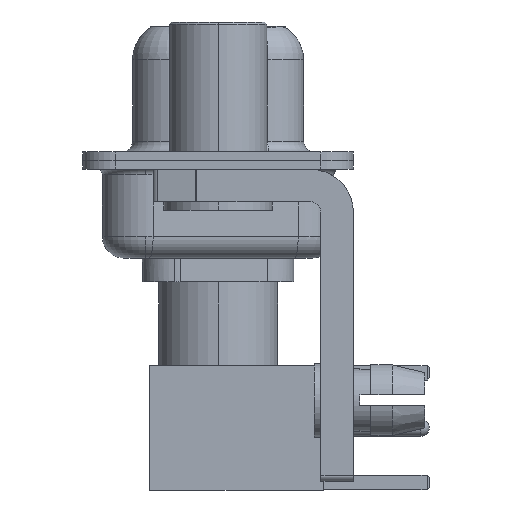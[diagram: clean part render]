
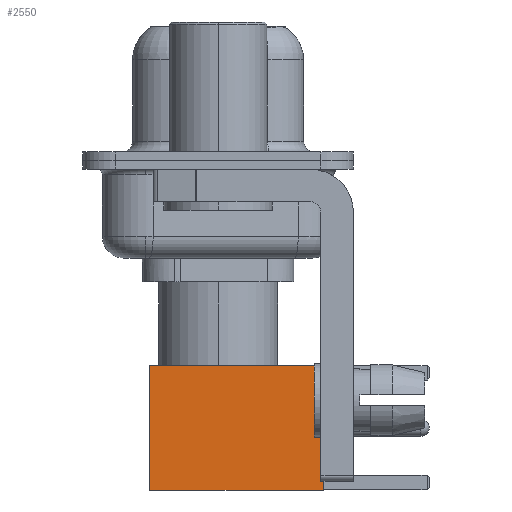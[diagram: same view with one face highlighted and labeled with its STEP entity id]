
A CAD part, left-side view. The second image highlights one B-rep face of the part: STEP entity #2550.
In plain terms, the highlighted face is planar.
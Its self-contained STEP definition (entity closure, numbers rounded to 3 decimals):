
#132 = VECTOR ( 'NONE', #5337, 1000. ) ;
#306 = VERTEX_POINT ( 'NONE', #8399 ) ;
#586 = DIRECTION ( 'NONE',  ( -1., 0., 0. ) ) ;
#611 = LINE ( 'NONE', #5249, #132 ) ;
#2097 = EDGE_CURVE ( 'NONE', #2786, #17092, #611, .T. ) ;
#2141 = PLANE ( 'NONE',  #15682 ) ;
#2550 = ADVANCED_FACE ( 'NONE', ( #15361 ), #2141, .T. ) ;
#2786 = VERTEX_POINT ( 'NONE', #10695 ) ;
#2857 = EDGE_LOOP ( 'NONE', ( #17352, #18047, #9110, #5099 ) ) ;
#3193 = VECTOR ( 'NONE', #18447, 1000. ) ;
#4827 = CARTESIAN_POINT ( 'NONE',  ( -2.875, 2.875, 8. ) ) ;
#5099 = ORIENTED_EDGE ( 'NONE', *, *, #9379, .F. ) ;
#5249 = CARTESIAN_POINT ( 'NONE',  ( 2.875, 2.875, 0. ) ) ;
#5337 = DIRECTION ( 'NONE',  ( 0., 0., -1. ) ) ;
#6705 = CARTESIAN_POINT ( 'NONE',  ( 2.875, 2.875, 0. ) ) ;
#8055 = CARTESIAN_POINT ( 'NONE',  ( 2.875, 2.875, 0. ) ) ;
#8399 = CARTESIAN_POINT ( 'NONE',  ( -2.875, 2.875, 0. ) ) ;
#8718 = LINE ( 'NONE', #8814, #17991 ) ;
#8814 = CARTESIAN_POINT ( 'NONE',  ( 0., 2.875, 0. ) ) ;
#9110 = ORIENTED_EDGE ( 'NONE', *, *, #9812, .F. ) ;
#9379 = EDGE_CURVE ( 'NONE', #2786, #11260, #18182, .T. ) ;
#9542 = EDGE_CURVE ( 'NONE', #17092, #306, #8718, .T. ) ;
#9587 = DIRECTION ( 'NONE',  ( 0., 1., 0. ) ) ;
#9812 = EDGE_CURVE ( 'NONE', #11260, #306, #16889, .T. ) ;
#10695 = CARTESIAN_POINT ( 'NONE',  ( 2.875, 2.875, 8. ) ) ;
#11260 = VERTEX_POINT ( 'NONE', #4827 ) ;
#13711 = CARTESIAN_POINT ( 'NONE',  ( -2.875, 2.875, 0. ) ) ;
#13924 = CARTESIAN_POINT ( 'NONE',  ( 0., 2.875, 8. ) ) ;
#14582 = DIRECTION ( 'NONE',  ( -1., 0., 0. ) ) ;
#15361 = FACE_OUTER_BOUND ( 'NONE', #2857, .T. ) ;
#15464 = DIRECTION ( 'NONE',  ( 0., 0., 1. ) ) ;
#15682 = AXIS2_PLACEMENT_3D ( 'NONE', #8055, #9587, #15464 ) ;
#16474 = VECTOR ( 'NONE', #586, 1000. ) ;
#16889 = LINE ( 'NONE', #13711, #3193 ) ;
#17092 = VERTEX_POINT ( 'NONE', #6705 ) ;
#17352 = ORIENTED_EDGE ( 'NONE', *, *, #2097, .T. ) ;
#17991 = VECTOR ( 'NONE', #14582, 1000. ) ;
#18047 = ORIENTED_EDGE ( 'NONE', *, *, #9542, .T. ) ;
#18182 = LINE ( 'NONE', #13924, #16474 ) ;
#18447 = DIRECTION ( 'NONE',  ( 0., 0., -1. ) ) ;
